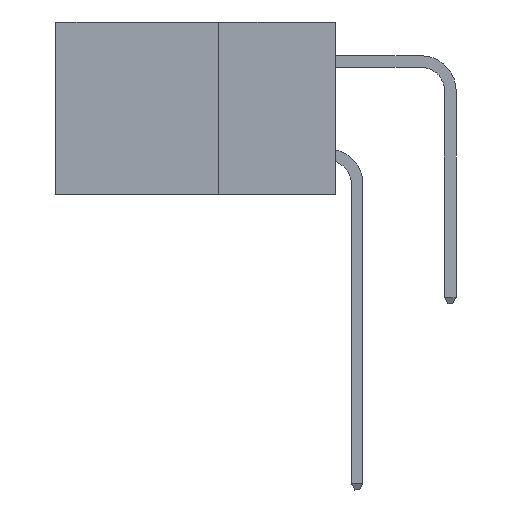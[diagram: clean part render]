
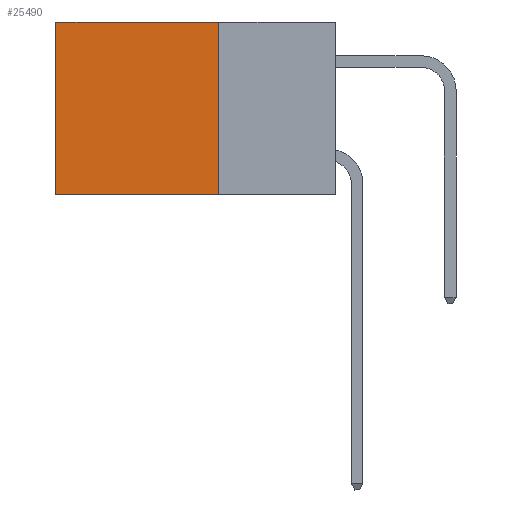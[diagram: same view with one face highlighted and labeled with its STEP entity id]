
A CAD part, left-side view. The second image highlights one B-rep face of the part: STEP entity #25490.
In plain terms, the highlighted planar face has unit normal (-1, 0, 0).
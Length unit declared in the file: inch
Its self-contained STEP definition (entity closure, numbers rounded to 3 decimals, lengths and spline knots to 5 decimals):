
#2690 = CARTESIAN_POINT ( 'NONE',  ( 0.2875, 0.25, -0.37 ) ) ;
#6129 = CARTESIAN_POINT ( 'NONE',  ( 0.2875, 0.25, 0. ) ) ;
#6238 = CARTESIAN_POINT ( 'NONE',  ( 0.2875, 0.25, 0. ) ) ;
#6950 = DIRECTION ( 'NONE',  ( 0., 0., -1. ) ) ;
#8508 = EDGE_CURVE ( 'NONE', #29182, #22288, #23121, .T. ) ;
#9882 = CARTESIAN_POINT ( 'NONE',  ( 0.2875, 0.25, -0.37 ) ) ;
#10498 = VECTOR ( 'NONE', #12800, 39.37008 ) ;
#10619 = DIRECTION ( 'NONE',  ( 0., 0., -1. ) ) ;
#11167 = CARTESIAN_POINT ( 'NONE',  ( 0.2875, 0.6, 0. ) ) ;
#11461 = VECTOR ( 'NONE', #22042, 39.37008 ) ;
#12800 = DIRECTION ( 'NONE',  ( 0., 1., 0. ) ) ;
#12958 = LINE ( 'NONE', #2690, #11461 ) ;
#14198 = VECTOR ( 'NONE', #6950, 39.37008 ) ;
#14544 = CARTESIAN_POINT ( 'NONE',  ( 0.2875, 0.6, 0. ) ) ;
#14943 = VERTEX_POINT ( 'NONE', #16893 ) ;
#15253 = EDGE_LOOP ( 'NONE', ( #25895, #32606, #36248, #34555 ) ) ;
#15270 = VERTEX_POINT ( 'NONE', #14544 ) ;
#16893 = CARTESIAN_POINT ( 'NONE',  ( 0.2875, 0.6, -0.37 ) ) ;
#18237 = DIRECTION ( 'NONE',  ( 1., 0., 0. ) ) ;
#20288 = AXIS2_PLACEMENT_3D ( 'NONE', #36765, #18237, #39989 ) ;
#20953 = VECTOR ( 'NONE', #10619, 39.37008 ) ;
#21218 = EDGE_CURVE ( 'NONE', #29182, #15270, #37787, .T. ) ;
#21585 = FACE_OUTER_BOUND ( 'NONE', #15253, .T. ) ;
#22042 = DIRECTION ( 'NONE',  ( 0., 1., 0. ) ) ;
#22288 = VERTEX_POINT ( 'NONE', #9882 ) ;
#23121 = LINE ( 'NONE', #29572, #14198 ) ;
#24218 = PLANE ( 'NONE',  #20288 ) ;
#25490 = ADVANCED_FACE ( 'NONE', ( #21585 ), #24218, .F. ) ;
#25895 = ORIENTED_EDGE ( 'NONE', *, *, #29910, .T. ) ;
#29182 = VERTEX_POINT ( 'NONE', #6129 ) ;
#29572 = CARTESIAN_POINT ( 'NONE',  ( 0.2875, 0.25, 0. ) ) ;
#29910 = EDGE_CURVE ( 'NONE', #15270, #14943, #38259, .T. ) ;
#32606 = ORIENTED_EDGE ( 'NONE', *, *, #36997, .F. ) ;
#34555 = ORIENTED_EDGE ( 'NONE', *, *, #21218, .T. ) ;
#36248 = ORIENTED_EDGE ( 'NONE', *, *, #8508, .F. ) ;
#36765 = CARTESIAN_POINT ( 'NONE',  ( 0.2875, 0.25, 0. ) ) ;
#36997 = EDGE_CURVE ( 'NONE', #22288, #14943, #12958, .T. ) ;
#37787 = LINE ( 'NONE', #6238, #10498 ) ;
#38259 = LINE ( 'NONE', #11167, #20953 ) ;
#39989 = DIRECTION ( 'NONE',  ( 0., 0., -1. ) ) ;
